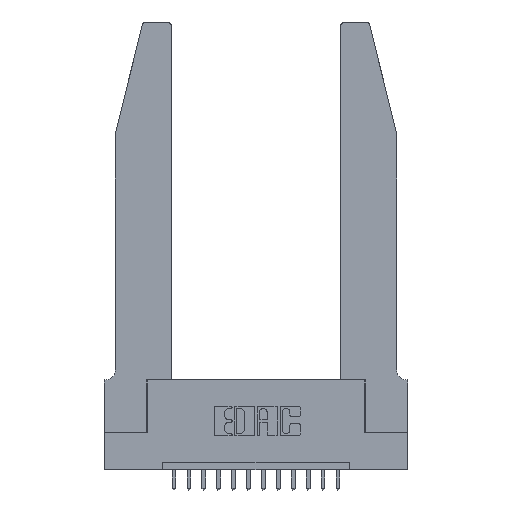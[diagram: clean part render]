
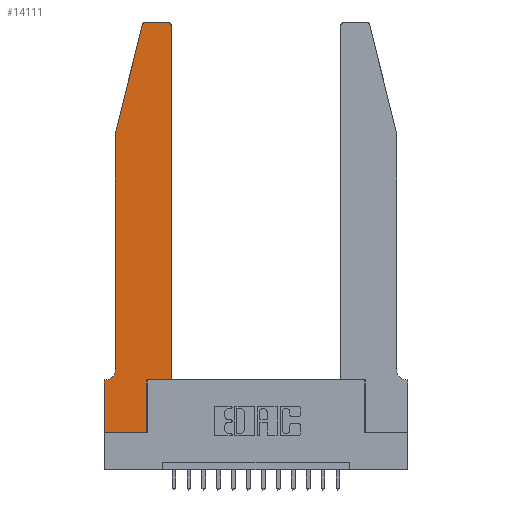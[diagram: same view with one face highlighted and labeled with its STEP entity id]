
A CAD part, top view. The second image highlights one B-rep face of the part: STEP entity #14111.
In plain terms, the highlighted planar face has unit normal (0, 0, 1).
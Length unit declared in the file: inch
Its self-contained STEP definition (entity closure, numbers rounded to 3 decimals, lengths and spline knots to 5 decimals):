
#86 = LINE ( 'NONE', #9624, #6804 ) ;
#275 = EDGE_LOOP ( 'NONE', ( #12192, #3881, #638, #2722, #17539, #8736, #12338, #10390, #17699, #7314, #10050, #837 ) ) ;
#633 = VERTEX_POINT ( 'NONE', #16604 ) ;
#638 = ORIENTED_EDGE ( 'NONE', *, *, #17798, .T. ) ;
#837 = ORIENTED_EDGE ( 'NONE', *, *, #9533, .T. ) ;
#871 = VERTEX_POINT ( 'NONE', #3428 ) ;
#1157 = VECTOR ( 'NONE', #2507, 39.37008 ) ;
#1397 = CARTESIAN_POINT ( 'NONE',  ( 0., 0.35, 0.37 ) ) ;
#1572 = VECTOR ( 'NONE', #14348, 39.37008 ) ;
#1575 = CARTESIAN_POINT ( 'NONE',  ( 0.0755, 2., 0.37 ) ) ;
#2208 = LINE ( 'NONE', #6583, #5032 ) ;
#2227 = AXIS2_PLACEMENT_3D ( 'NONE', #11875, #14614, #16006 ) ;
#2342 = VERTEX_POINT ( 'NONE', #16541 ) ;
#2449 = CARTESIAN_POINT ( 'NONE',  ( 0., 0., 0.37 ) ) ;
#2507 = DIRECTION ( 'NONE',  ( 0., -1., 0. ) ) ;
#2722 = ORIENTED_EDGE ( 'NONE', *, *, #8229, .T. ) ;
#2745 = VERTEX_POINT ( 'NONE', #10472 ) ;
#2845 = CARTESIAN_POINT ( 'NONE',  ( 0.4205, 2.75, 0.37 ) ) ;
#2885 = EDGE_CURVE ( 'NONE', #871, #9028, #16091, .T. ) ;
#3336 = CIRCLE ( 'NONE', #13116, 0.07 ) ;
#3419 = CARTESIAN_POINT ( 'NONE',  ( 0.0755, 2., 0.37 ) ) ;
#3428 = CARTESIAN_POINT ( 'NONE',  ( 0., 0., 0.37 ) ) ;
#3495 = CIRCLE ( 'NONE', #2227, 0.03 ) ;
#3547 = LINE ( 'NONE', #3419, #1572 ) ;
#3601 = VECTOR ( 'NONE', #7305, 39.37008 ) ;
#3881 = ORIENTED_EDGE ( 'NONE', *, *, #17134, .T. ) ;
#4067 = AXIS2_PLACEMENT_3D ( 'NONE', #4353, #4480, #13901 ) ;
#4138 = AXIS2_PLACEMENT_3D ( 'NONE', #1397, #13757, #12315 ) ;
#4353 = CARTESIAN_POINT ( 'NONE',  ( 0.284, 2.72, 0.37 ) ) ;
#4480 = DIRECTION ( 'NONE',  ( 0., 0., 1. ) ) ;
#4618 = VERTEX_POINT ( 'NONE', #7583 ) ;
#4713 = VECTOR ( 'NONE', #14803, 39.37008 ) ;
#5032 = VECTOR ( 'NONE', #17524, 39.37008 ) ;
#5050 = CARTESIAN_POINT ( 'NONE',  ( 0.25487, 2.72718, 0.37 ) ) ;
#5085 = CARTESIAN_POINT ( 'NONE',  ( 0.2865, 0., 0.37 ) ) ;
#5097 = CARTESIAN_POINT ( 'NONE',  ( 0.0055, 0.42, 0.37 ) ) ;
#5815 = DIRECTION ( 'NONE',  ( 0., -1., 0. ) ) ;
#6573 = VERTEX_POINT ( 'NONE', #7362 ) ;
#6583 = CARTESIAN_POINT ( 'NONE',  ( 0.2865, 0.35, 0.37 ) ) ;
#6694 = DIRECTION ( 'NONE',  ( 1., 0., 0. ) ) ;
#6766 = LINE ( 'NONE', #1575, #8899 ) ;
#6804 = VECTOR ( 'NONE', #8185, 39.37008 ) ;
#6848 = CARTESIAN_POINT ( 'NONE',  ( 0.284, 2.75, 0.37 ) ) ;
#7305 = DIRECTION ( 'NONE',  ( 0., 1., 0. ) ) ;
#7314 = ORIENTED_EDGE ( 'NONE', *, *, #14565, .T. ) ;
#7362 = CARTESIAN_POINT ( 'NONE',  ( 0.2865, 0.35, 0.37 ) ) ;
#7448 = VERTEX_POINT ( 'NONE', #6848 ) ;
#7583 = CARTESIAN_POINT ( 'NONE',  ( 0.0755, 2., 0.37 ) ) ;
#8185 = DIRECTION ( 'NONE',  ( -1., 0., 0. ) ) ;
#8229 = EDGE_CURVE ( 'NONE', #4618, #11002, #6766, .T. ) ;
#8299 = CARTESIAN_POINT ( 'NONE',  ( 0., 0., 0.37 ) ) ;
#8736 = ORIENTED_EDGE ( 'NONE', *, *, #16983, .T. ) ;
#8748 = CARTESIAN_POINT ( 'NONE',  ( 0.4505, 0.35, 0.37 ) ) ;
#8899 = VECTOR ( 'NONE', #5815, 39.37008 ) ;
#9028 = VERTEX_POINT ( 'NONE', #5085 ) ;
#9516 = LINE ( 'NONE', #15808, #11020 ) ;
#9533 = EDGE_CURVE ( 'NONE', #2745, #10332, #3495, .T. ) ;
#9578 = CIRCLE ( 'NONE', #4067, 0.03 ) ;
#9624 = CARTESIAN_POINT ( 'NONE',  ( 0.0755, 0.35, 0.37 ) ) ;
#10050 = ORIENTED_EDGE ( 'NONE', *, *, #15486, .T. ) ;
#10332 = VERTEX_POINT ( 'NONE', #2845 ) ;
#10390 = ORIENTED_EDGE ( 'NONE', *, *, #2885, .T. ) ;
#10472 = CARTESIAN_POINT ( 'NONE',  ( 0.4505, 2.72, 0.37 ) ) ;
#11002 = VERTEX_POINT ( 'NONE', #16094 ) ;
#11020 = VECTOR ( 'NONE', #13371, 39.37008 ) ;
#11602 = EDGE_CURVE ( 'NONE', #9028, #6573, #2208, .T. ) ;
#11875 = CARTESIAN_POINT ( 'NONE',  ( 0.4205, 2.72, 0.37 ) ) ;
#12022 = VECTOR ( 'NONE', #6694, 39.37008 ) ;
#12029 = LINE ( 'NONE', #13435, #4713 ) ;
#12192 = ORIENTED_EDGE ( 'NONE', *, *, #12221, .T. ) ;
#12221 = EDGE_CURVE ( 'NONE', #10332, #7448, #9516, .T. ) ;
#12315 = DIRECTION ( 'NONE',  ( 1., 0., 0. ) ) ;
#12338 = ORIENTED_EDGE ( 'NONE', *, *, #16874, .T. ) ;
#12369 = PLANE ( 'NONE',  #4138 ) ;
#12720 = VERTEX_POINT ( 'NONE', #14505 ) ;
#13116 = AXIS2_PLACEMENT_3D ( 'NONE', #5097, #14688, #16083 ) ;
#13371 = DIRECTION ( 'NONE',  ( -1., 0., 0. ) ) ;
#13435 = CARTESIAN_POINT ( 'NONE',  ( 0.4505, 0.35, 0.37 ) ) ;
#13593 = VERTEX_POINT ( 'NONE', #5050 ) ;
#13757 = DIRECTION ( 'NONE',  ( 0., 0., 1. ) ) ;
#13901 = DIRECTION ( 'NONE',  ( 1., 0., 0. ) ) ;
#14111 = ADVANCED_FACE ( 'NONE', ( #14386 ), #12369, .T. ) ;
#14348 = DIRECTION ( 'NONE',  ( -0.239, -0.971, 0. ) ) ;
#14386 = FACE_OUTER_BOUND ( 'NONE', #275, .T. ) ;
#14505 = CARTESIAN_POINT ( 'NONE',  ( 0.0055, 0.35, 0.37 ) ) ;
#14565 = EDGE_CURVE ( 'NONE', #6573, #633, #12029, .T. ) ;
#14614 = DIRECTION ( 'NONE',  ( 0., 0., 1. ) ) ;
#14688 = DIRECTION ( 'NONE',  ( 0., 0., -1. ) ) ;
#14803 = DIRECTION ( 'NONE',  ( 1., 0., 0. ) ) ;
#15381 = LINE ( 'NONE', #2449, #1157 ) ;
#15486 = EDGE_CURVE ( 'NONE', #633, #2745, #17792, .T. ) ;
#15808 = CARTESIAN_POINT ( 'NONE',  ( 0.2605, 2.75, 0.37 ) ) ;
#16006 = DIRECTION ( 'NONE',  ( 1., 0., 0. ) ) ;
#16083 = DIRECTION ( 'NONE',  ( -1., 0., 0. ) ) ;
#16091 = LINE ( 'NONE', #8299, #12022 ) ;
#16094 = CARTESIAN_POINT ( 'NONE',  ( 0.0755, 0.42, 0.37 ) ) ;
#16256 = EDGE_CURVE ( 'NONE', #11002, #12720, #3336, .T. ) ;
#16541 = CARTESIAN_POINT ( 'NONE',  ( 0., 0.35, 0.37 ) ) ;
#16604 = CARTESIAN_POINT ( 'NONE',  ( 0.4505, 0.35, 0.37 ) ) ;
#16874 = EDGE_CURVE ( 'NONE', #2342, #871, #15381, .T. ) ;
#16983 = EDGE_CURVE ( 'NONE', #12720, #2342, #86, .T. ) ;
#17134 = EDGE_CURVE ( 'NONE', #7448, #13593, #9578, .T. ) ;
#17524 = DIRECTION ( 'NONE',  ( 0., 1., 0. ) ) ;
#17539 = ORIENTED_EDGE ( 'NONE', *, *, #16256, .T. ) ;
#17699 = ORIENTED_EDGE ( 'NONE', *, *, #11602, .T. ) ;
#17792 = LINE ( 'NONE', #8748, #3601 ) ;
#17798 = EDGE_CURVE ( 'NONE', #13593, #4618, #3547, .T. ) ;
